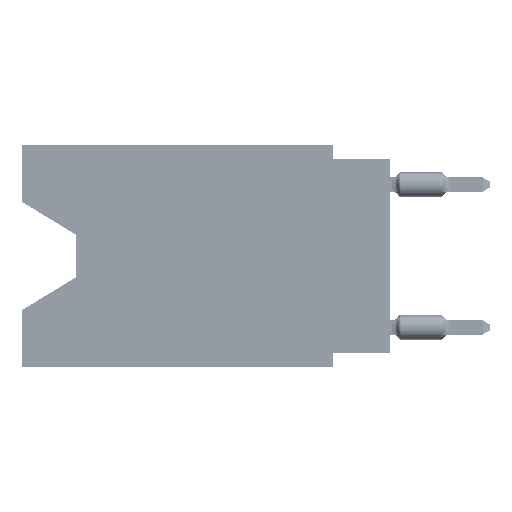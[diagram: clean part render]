
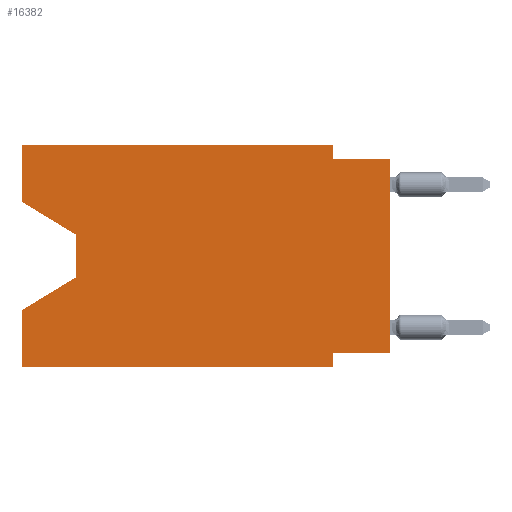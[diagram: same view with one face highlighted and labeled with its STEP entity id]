
A CAD part, left-side view. The second image highlights one B-rep face of the part: STEP entity #16382.
In plain terms, the highlighted planar face has unit normal (-1, 0, 0).
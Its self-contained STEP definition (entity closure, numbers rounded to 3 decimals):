
#31 = DIRECTION ( 'NONE',  ( 0., -1., 0. ) ) ;
#534 = CARTESIAN_POINT ( 'NONE',  ( 0., 16.383, -7.36 ) ) ;
#983 = ORIENTED_EDGE ( 'NONE', *, *, #60918, .T. ) ;
#1793 = CARTESIAN_POINT ( 'NONE',  ( 0., 16.383, 0. ) ) ;
#2088 = LINE ( 'NONE', #32032, #13964 ) ;
#2136 = ORIENTED_EDGE ( 'NONE', *, *, #74532, .F. ) ;
#2492 = VERTEX_POINT ( 'NONE', #23809 ) ;
#3675 = CARTESIAN_POINT ( 'NONE',  ( 0., 0., -0.635 ) ) ;
#5142 = CARTESIAN_POINT ( 'NONE',  ( 0., 2.54, -9.906 ) ) ;
#5508 = EDGE_CURVE ( 'NONE', #17888, #68831, #38444, .T. ) ;
#7413 = VERTEX_POINT ( 'NONE', #9017 ) ;
#8044 = DIRECTION ( 'NONE',  ( 0., 0., -1. ) ) ;
#9017 = CARTESIAN_POINT ( 'NONE',  ( 0., 13.97, -4.013 ) ) ;
#10664 = AXIS2_PLACEMENT_3D ( 'NONE', #46955, #40971, #76058 ) ;
#11154 = ORIENTED_EDGE ( 'NONE', *, *, #38232, .T. ) ;
#12737 = LINE ( 'NONE', #47892, #43516 ) ;
#13504 = ORIENTED_EDGE ( 'NONE', *, *, #35931, .F. ) ;
#13964 = VECTOR ( 'NONE', #44021, 1000. ) ;
#14440 = CARTESIAN_POINT ( 'NONE',  ( 0., 0., -9.271 ) ) ;
#15423 = EDGE_CURVE ( 'NONE', #37983, #28651, #75452, .T. ) ;
#16382 = ADVANCED_FACE ( 'NONE', ( #63711 ), #46561, .F. ) ;
#16716 = CARTESIAN_POINT ( 'NONE',  ( 0., 16.383, -2.546 ) ) ;
#17888 = VERTEX_POINT ( 'NONE', #16716 ) ;
#18638 = DIRECTION ( 'NONE',  ( 0., 0., 1. ) ) ;
#18903 = CARTESIAN_POINT ( 'NONE',  ( 0., 16.383, 0. ) ) ;
#18916 = DIRECTION ( 'NONE',  ( 0., 0., -1. ) ) ;
#19753 = VERTEX_POINT ( 'NONE', #20168 ) ;
#20168 = CARTESIAN_POINT ( 'NONE',  ( 0., 2.54, 0. ) ) ;
#22835 = VECTOR ( 'NONE', #62782, 1000. ) ;
#23809 = CARTESIAN_POINT ( 'NONE',  ( 0., 2.54, -0.635 ) ) ;
#24624 = EDGE_CURVE ( 'NONE', #28651, #71087, #45535, .T. ) ;
#25584 = LINE ( 'NONE', #43159, #67539 ) ;
#26047 = ORIENTED_EDGE ( 'NONE', *, *, #47741, .F. ) ;
#26874 = CARTESIAN_POINT ( 'NONE',  ( 0., 13.97, -4.013 ) ) ;
#27401 = LINE ( 'NONE', #45736, #56390 ) ;
#28061 = LINE ( 'NONE', #26874, #70034 ) ;
#28651 = VERTEX_POINT ( 'NONE', #63093 ) ;
#29274 = CARTESIAN_POINT ( 'NONE',  ( 0., 0., 0. ) ) ;
#30475 = VECTOR ( 'NONE', #8044, 1000. ) ;
#31636 = VECTOR ( 'NONE', #71144, 1000. ) ;
#31993 = CARTESIAN_POINT ( 'NONE',  ( 0., 2.54, -9.906 ) ) ;
#32032 = CARTESIAN_POINT ( 'NONE',  ( 0., 16.383, -2.546 ) ) ;
#34344 = ORIENTED_EDGE ( 'NONE', *, *, #15423, .F. ) ;
#35707 = CARTESIAN_POINT ( 'NONE',  ( 0., 2.54, 0. ) ) ;
#35916 = DIRECTION ( 'NONE',  ( 0., -1., 0. ) ) ;
#35931 = EDGE_CURVE ( 'NONE', #68831, #19753, #61855, .T. ) ;
#37983 = VERTEX_POINT ( 'NONE', #68795 ) ;
#38175 = ORIENTED_EDGE ( 'NONE', *, *, #24624, .F. ) ;
#38232 = EDGE_CURVE ( 'NONE', #37983, #60030, #41643, .T. ) ;
#38444 = LINE ( 'NONE', #18903, #22835 ) ;
#39612 = EDGE_CURVE ( 'NONE', #17888, #7413, #2088, .T. ) ;
#40971 = DIRECTION ( 'NONE',  ( 1., 0., 0. ) ) ;
#41166 = VERTEX_POINT ( 'NONE', #534 ) ;
#41643 = LINE ( 'NONE', #29274, #31636 ) ;
#42192 = CARTESIAN_POINT ( 'NONE',  ( 0., 16.383, 0. ) ) ;
#43159 = CARTESIAN_POINT ( 'NONE',  ( 0., 16.383, -9.906 ) ) ;
#43516 = VECTOR ( 'NONE', #35916, 1000. ) ;
#44011 = DIRECTION ( 'NONE',  ( 0., 1., 0. ) ) ;
#44021 = DIRECTION ( 'NONE',  ( 0., -0.855, -0.519 ) ) ;
#44047 = VECTOR ( 'NONE', #18916, 1000. ) ;
#45535 = LINE ( 'NONE', #31993, #30475 ) ;
#45736 = CARTESIAN_POINT ( 'NONE',  ( 0., 13.97, -5.893 ) ) ;
#46123 = DIRECTION ( 'NONE',  ( 0., 0.855, -0.519 ) ) ;
#46561 = PLANE ( 'NONE',  #10664 ) ;
#46955 = CARTESIAN_POINT ( 'NONE',  ( 0., 16.383, 0. ) ) ;
#47741 = EDGE_CURVE ( 'NONE', #19753, #2492, #61195, .T. ) ;
#47892 = CARTESIAN_POINT ( 'NONE',  ( 0., 0., -0.635 ) ) ;
#48630 = EDGE_CURVE ( 'NONE', #58205, #41166, #73275, .T. ) ;
#49885 = DIRECTION ( 'NONE',  ( 0., -1., 0. ) ) ;
#50294 = VECTOR ( 'NONE', #18638, 1000. ) ;
#50541 = ORIENTED_EDGE ( 'NONE', *, *, #5508, .F. ) ;
#52382 = DIRECTION ( 'NONE',  ( 0., 0., -1. ) ) ;
#52593 = VECTOR ( 'NONE', #44011, 1000. ) ;
#54365 = EDGE_CURVE ( 'NONE', #58308, #41166, #27401, .T. ) ;
#55065 = CARTESIAN_POINT ( 'NONE',  ( 0., 16.383, 0. ) ) ;
#56390 = VECTOR ( 'NONE', #46123, 1000. ) ;
#58205 = VERTEX_POINT ( 'NONE', #68820 ) ;
#58308 = VERTEX_POINT ( 'NONE', #65191 ) ;
#60030 = VERTEX_POINT ( 'NONE', #3675 ) ;
#60235 = ORIENTED_EDGE ( 'NONE', *, *, #48630, .F. ) ;
#60918 = EDGE_CURVE ( 'NONE', #58205, #71087, #25584, .T. ) ;
#61195 = LINE ( 'NONE', #35707, #44047 ) ;
#61855 = LINE ( 'NONE', #55065, #67021 ) ;
#61928 = EDGE_CURVE ( 'NONE', #7413, #58308, #28061, .T. ) ;
#62625 = ORIENTED_EDGE ( 'NONE', *, *, #54365, .T. ) ;
#62782 = DIRECTION ( 'NONE',  ( 0., 0., 1. ) ) ;
#63093 = CARTESIAN_POINT ( 'NONE',  ( 0., 2.54, -9.271 ) ) ;
#63711 = FACE_OUTER_BOUND ( 'NONE', #75509, .T. ) ;
#65191 = CARTESIAN_POINT ( 'NONE',  ( 0., 13.97, -5.893 ) ) ;
#65545 = ORIENTED_EDGE ( 'NONE', *, *, #61928, .T. ) ;
#67021 = VECTOR ( 'NONE', #49885, 1000. ) ;
#67539 = VECTOR ( 'NONE', #31, 1000. ) ;
#68795 = CARTESIAN_POINT ( 'NONE',  ( 0., 0., -9.271 ) ) ;
#68820 = CARTESIAN_POINT ( 'NONE',  ( 0., 16.383, -9.906 ) ) ;
#68831 = VERTEX_POINT ( 'NONE', #1793 ) ;
#70034 = VECTOR ( 'NONE', #52382, 1000. ) ;
#71087 = VERTEX_POINT ( 'NONE', #5142 ) ;
#71144 = DIRECTION ( 'NONE',  ( 0., 0., 1. ) ) ;
#72554 = ORIENTED_EDGE ( 'NONE', *, *, #39612, .T. ) ;
#73275 = LINE ( 'NONE', #42192, #50294 ) ;
#74532 = EDGE_CURVE ( 'NONE', #2492, #60030, #12737, .T. ) ;
#75452 = LINE ( 'NONE', #14440, #52593 ) ;
#75509 = EDGE_LOOP ( 'NONE', ( #72554, #65545, #62625, #60235, #983, #38175, #34344, #11154, #2136, #26047, #13504, #50541 ) ) ;
#76058 = DIRECTION ( 'NONE',  ( 0., 0., -1. ) ) ;
